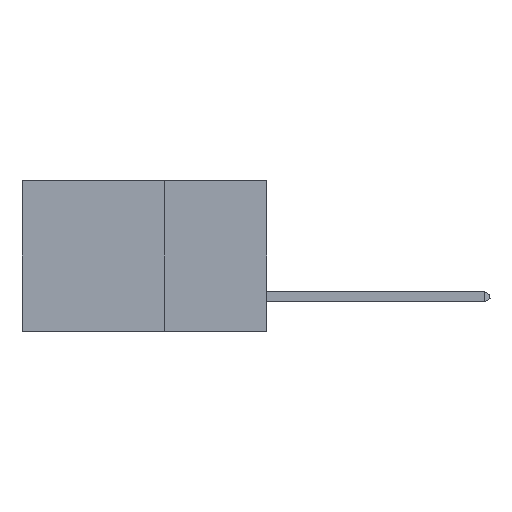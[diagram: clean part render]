
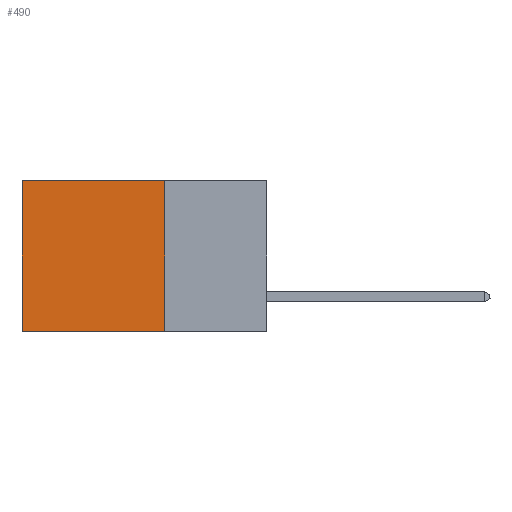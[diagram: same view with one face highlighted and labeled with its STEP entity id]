
A CAD part, left-side view. The second image highlights one B-rep face of the part: STEP entity #490.
In plain terms, the highlighted planar face has unit normal (-1, 0, 0).
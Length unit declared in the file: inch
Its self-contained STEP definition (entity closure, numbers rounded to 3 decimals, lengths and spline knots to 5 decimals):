
#96 = LINE ( 'NONE', #5728, #5305 ) ;
#428 = DIRECTION ( 'NONE',  ( 1., 0., 0. ) ) ;
#490 = ADVANCED_FACE ( 'NONE', ( #4833 ), #9584, .F. ) ;
#706 = CARTESIAN_POINT ( 'NONE',  ( 0.2875, 0.25, -0.37 ) ) ;
#1264 = CARTESIAN_POINT ( 'NONE',  ( 0.2875, 0.25, 0. ) ) ;
#1673 = DIRECTION ( 'NONE',  ( 0., 0., -1. ) ) ;
#1918 = LINE ( 'NONE', #10899, #12649 ) ;
#2945 = ORIENTED_EDGE ( 'NONE', *, *, #10180, .F. ) ;
#3237 = EDGE_LOOP ( 'NONE', ( #9945, #7087, #2945, #5309 ) ) ;
#3487 = VERTEX_POINT ( 'NONE', #10978 ) ;
#3541 = EDGE_CURVE ( 'NONE', #5547, #3487, #1918, .T. ) ;
#3715 = VECTOR ( 'NONE', #4415, 39.37008 ) ;
#3780 = CARTESIAN_POINT ( 'NONE',  ( 0.2875, 0.6, 0. ) ) ;
#3920 = DIRECTION ( 'NONE',  ( 0., 0., -1. ) ) ;
#4344 = VECTOR ( 'NONE', #9231, 39.37008 ) ;
#4415 = DIRECTION ( 'NONE',  ( 0., 1., 0. ) ) ;
#4833 = FACE_OUTER_BOUND ( 'NONE', #3237, .T. ) ;
#5022 = VERTEX_POINT ( 'NONE', #706 ) ;
#5305 = VECTOR ( 'NONE', #1673, 39.37008 ) ;
#5309 = ORIENTED_EDGE ( 'NONE', *, *, #7823, .T. ) ;
#5547 = VERTEX_POINT ( 'NONE', #3780 ) ;
#5728 = CARTESIAN_POINT ( 'NONE',  ( 0.2875, 0.25, 0. ) ) ;
#7087 = ORIENTED_EDGE ( 'NONE', *, *, #7708, .F. ) ;
#7177 = VERTEX_POINT ( 'NONE', #8075 ) ;
#7627 = LINE ( 'NONE', #10074, #4344 ) ;
#7708 = EDGE_CURVE ( 'NONE', #5022, #3487, #7627, .T. ) ;
#7823 = EDGE_CURVE ( 'NONE', #7177, #5547, #9548, .T. ) ;
#8075 = CARTESIAN_POINT ( 'NONE',  ( 0.2875, 0.25, 0. ) ) ;
#8359 = DIRECTION ( 'NONE',  ( 0., 0., -1. ) ) ;
#9231 = DIRECTION ( 'NONE',  ( 0., 1., 0. ) ) ;
#9548 = LINE ( 'NONE', #1264, #3715 ) ;
#9584 = PLANE ( 'NONE',  #9722 ) ;
#9722 = AXIS2_PLACEMENT_3D ( 'NONE', #10582, #428, #8359 ) ;
#9945 = ORIENTED_EDGE ( 'NONE', *, *, #3541, .T. ) ;
#10074 = CARTESIAN_POINT ( 'NONE',  ( 0.2875, 0.25, -0.37 ) ) ;
#10180 = EDGE_CURVE ( 'NONE', #7177, #5022, #96, .T. ) ;
#10582 = CARTESIAN_POINT ( 'NONE',  ( 0.2875, 0.25, 0. ) ) ;
#10899 = CARTESIAN_POINT ( 'NONE',  ( 0.2875, 0.6, 0. ) ) ;
#10978 = CARTESIAN_POINT ( 'NONE',  ( 0.2875, 0.6, -0.37 ) ) ;
#12649 = VECTOR ( 'NONE', #3920, 39.37008 ) ;
